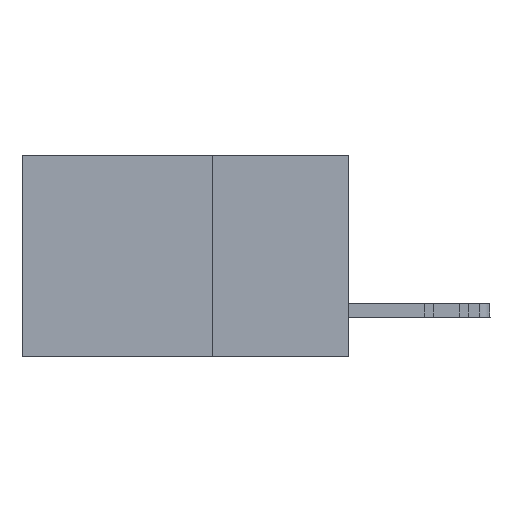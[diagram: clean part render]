
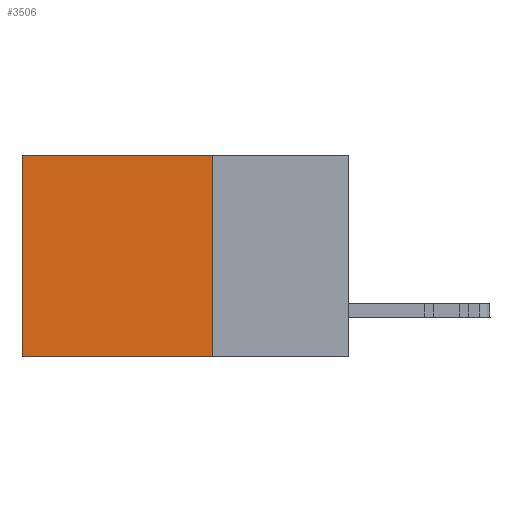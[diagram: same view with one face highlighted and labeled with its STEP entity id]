
A CAD part, left-side view. The second image highlights one B-rep face of the part: STEP entity #3506.
In plain terms, the highlighted planar face has unit normal (-1, 0, 0).
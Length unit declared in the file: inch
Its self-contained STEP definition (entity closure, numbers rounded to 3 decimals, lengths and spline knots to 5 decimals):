
#390 = CARTESIAN_POINT ( 'NONE',  ( 0.298, 0.6, 0. ) ) ;
#527 = ORIENTED_EDGE ( 'NONE', *, *, #16642, .T. ) ;
#575 = VECTOR ( 'NONE', #17306, 39.37008 ) ;
#1388 = CARTESIAN_POINT ( 'NONE',  ( 0.298, 0.25, 0. ) ) ;
#1794 = VERTEX_POINT ( 'NONE', #26025 ) ;
#2780 = AXIS2_PLACEMENT_3D ( 'NONE', #1388, #5838, #14318 ) ;
#3506 = ADVANCED_FACE ( 'NONE', ( #22691 ), #20733, .F. ) ;
#4039 = CARTESIAN_POINT ( 'NONE',  ( 0.298, 0.25, -0.37 ) ) ;
#4119 = ORIENTED_EDGE ( 'NONE', *, *, #12889, .T. ) ;
#4958 = DIRECTION ( 'NONE',  ( 0., 0., -1. ) ) ;
#5091 = EDGE_CURVE ( 'NONE', #1794, #27161, #23110, .T. ) ;
#5257 = ORIENTED_EDGE ( 'NONE', *, *, #14236, .F. ) ;
#5838 = DIRECTION ( 'NONE',  ( 1., 0., 0. ) ) ;
#9348 = CARTESIAN_POINT ( 'NONE',  ( 0.298, 0.25, 0. ) ) ;
#9443 = VERTEX_POINT ( 'NONE', #25163 ) ;
#9994 = CARTESIAN_POINT ( 'NONE',  ( 0.298, 0.6, -0.37 ) ) ;
#10574 = CARTESIAN_POINT ( 'NONE',  ( 0.298, 0.25, 0. ) ) ;
#11188 = ORIENTED_EDGE ( 'NONE', *, *, #5091, .F. ) ;
#12797 = CARTESIAN_POINT ( 'NONE',  ( 0.298, 0.25, 0. ) ) ;
#12889 = EDGE_CURVE ( 'NONE', #9443, #27161, #23763, .T. ) ;
#14236 = EDGE_CURVE ( 'NONE', #18802, #1794, #23396, .T. ) ;
#14318 = DIRECTION ( 'NONE',  ( 0., 0., -1. ) ) ;
#16642 = EDGE_CURVE ( 'NONE', #18802, #9443, #21630, .T. ) ;
#17306 = DIRECTION ( 'NONE',  ( 0., 1., 0. ) ) ;
#18802 = VERTEX_POINT ( 'NONE', #10574 ) ;
#19202 = DIRECTION ( 'NONE',  ( 0., 0., -1. ) ) ;
#20733 = PLANE ( 'NONE',  #2780 ) ;
#21159 = DIRECTION ( 'NONE',  ( 0., 1., 0. ) ) ;
#21630 = LINE ( 'NONE', #9348, #575 ) ;
#21822 = VECTOR ( 'NONE', #19202, 39.37008 ) ;
#22691 = FACE_OUTER_BOUND ( 'NONE', #22868, .T. ) ;
#22868 = EDGE_LOOP ( 'NONE', ( #4119, #11188, #5257, #527 ) ) ;
#23110 = LINE ( 'NONE', #4039, #25940 ) ;
#23396 = LINE ( 'NONE', #12797, #21822 ) ;
#23763 = LINE ( 'NONE', #390, #24438 ) ;
#24438 = VECTOR ( 'NONE', #4958, 39.37008 ) ;
#25163 = CARTESIAN_POINT ( 'NONE',  ( 0.298, 0.6, 0. ) ) ;
#25940 = VECTOR ( 'NONE', #21159, 39.37008 ) ;
#26025 = CARTESIAN_POINT ( 'NONE',  ( 0.298, 0.25, -0.37 ) ) ;
#27161 = VERTEX_POINT ( 'NONE', #9994 ) ;
